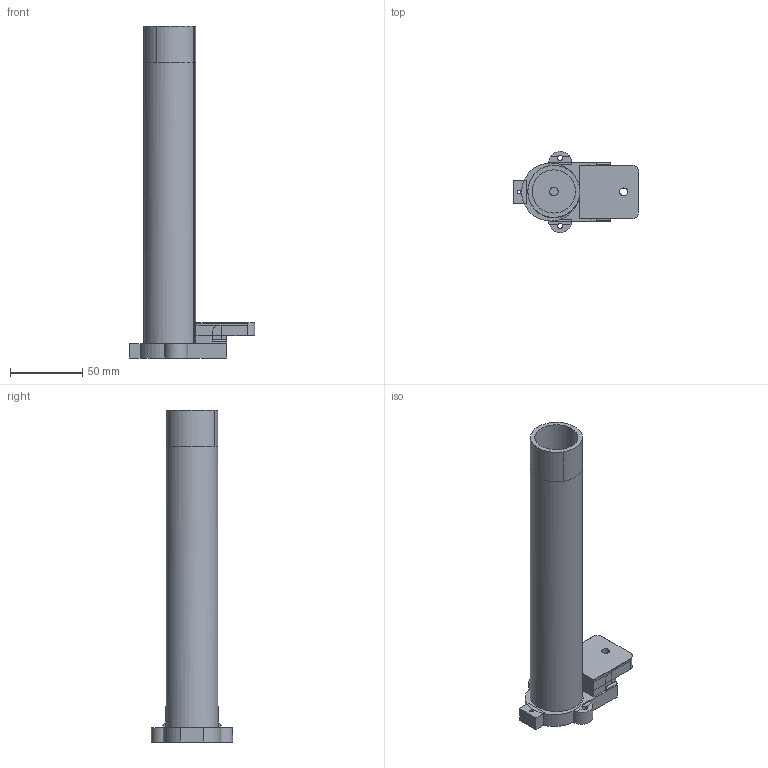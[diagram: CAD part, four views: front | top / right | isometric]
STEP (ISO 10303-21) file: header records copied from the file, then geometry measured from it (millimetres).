
FILE_DESCRIPTION(('FreeCAD Model'),'2;1');
FILE_NAME('ap9 buffer tube 2020.step','2020-04-04T17:42:10',('Author'),(''), 'Open CASCADE STEP processor 6.8','FreeCAD','Unknown');
FILE_SCHEMA(('AUTOMOTIVE_DESIGN_CC2 { 1 2 10303 214 -1 1 5 4 }'));
Length unit declared in the file: millimetre
Products named in the file (1): Pocket
Bounding box: 86.94 x 56.2 x 230 mm (x, y, z)
Volume: 155822.6 mm3; surface area: 53327.1 mm2
Topology: 1 solids, 1 shells, 105 faces, 265 edges, 166 vertices
Faces by surface type: plane 76, cylinder 28, bspline 1
Full cylindrical faces by diameter (mm): 2.4 x1, 3.7 x2, 5.5 x1, 17.93 x1, 26 x1, 30 x2
Entity records: 6923 total; most frequent: CARTESIAN_POINT 1644, DIRECTION 998, LINE 572, VECTOR 572, ORIENTED_EDGE 530, PCURVE 530, DEFINITIONAL_REPRESENTATION 530, EDGE_CURVE 265
